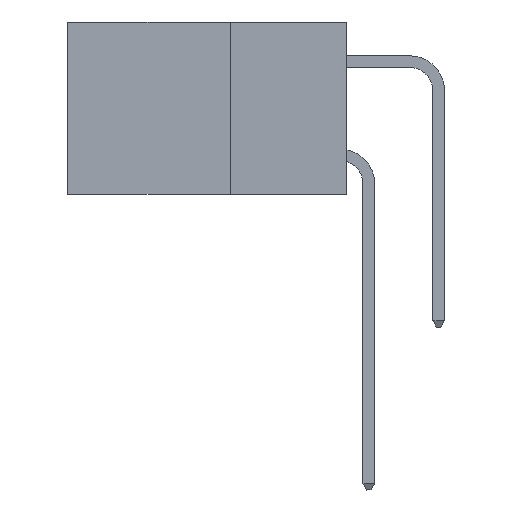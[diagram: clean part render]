
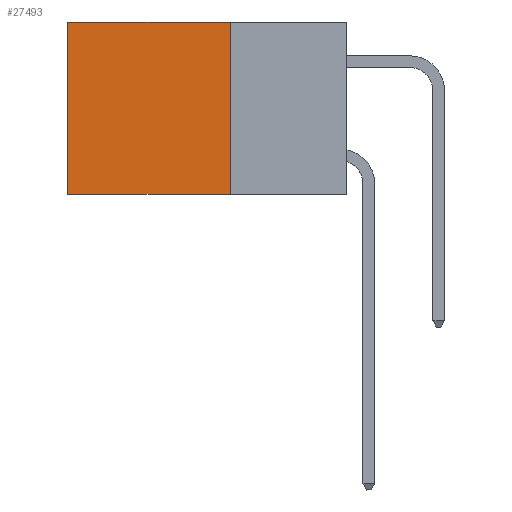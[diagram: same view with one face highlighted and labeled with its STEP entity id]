
A CAD part, left-side view. The second image highlights one B-rep face of the part: STEP entity #27493.
In plain terms, the highlighted planar face has unit normal (-1, 0, 0).
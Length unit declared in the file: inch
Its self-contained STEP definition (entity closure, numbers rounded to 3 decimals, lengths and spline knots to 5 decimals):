
#363 = VERTEX_POINT ( 'NONE', #18984 ) ;
#1046 = DIRECTION ( 'NONE',  ( 0., 1., 0. ) ) ;
#2735 = CARTESIAN_POINT ( 'NONE',  ( 0.2875, 0.25, -0.37 ) ) ;
#2800 = DIRECTION ( 'NONE',  ( 0., 0., -1. ) ) ;
#3323 = VERTEX_POINT ( 'NONE', #14393 ) ;
#4624 = EDGE_CURVE ( 'NONE', #3323, #363, #29735, .T. ) ;
#5060 = ORIENTED_EDGE ( 'NONE', *, *, #22631, .F. ) ;
#7371 = VECTOR ( 'NONE', #22149, 39.37008 ) ;
#7575 = ORIENTED_EDGE ( 'NONE', *, *, #4624, .T. ) ;
#7855 = LINE ( 'NONE', #24514, #26828 ) ;
#8529 = CARTESIAN_POINT ( 'NONE',  ( 0.2875, 0.25, 0. ) ) ;
#8904 = DIRECTION ( 'NONE',  ( 0., 0., -1. ) ) ;
#9681 = FACE_OUTER_BOUND ( 'NONE', #22427, .T. ) ;
#9846 = AXIS2_PLACEMENT_3D ( 'NONE', #18028, #20456, #2800 ) ;
#13505 = EDGE_CURVE ( 'NONE', #3323, #29063, #32188, .T. ) ;
#14393 = CARTESIAN_POINT ( 'NONE',  ( 0.2875, 0.25, 0. ) ) ;
#15270 = ORIENTED_EDGE ( 'NONE', *, *, #13505, .F. ) ;
#15815 = PLANE ( 'NONE',  #9846 ) ;
#16532 = CARTESIAN_POINT ( 'NONE',  ( 0.2875, 0.25, 0. ) ) ;
#17319 = EDGE_CURVE ( 'NONE', #363, #26262, #7855, .T. ) ;
#18028 = CARTESIAN_POINT ( 'NONE',  ( 0.2875, 0.25, 0. ) ) ;
#18984 = CARTESIAN_POINT ( 'NONE',  ( 0.2875, 0.6, 0. ) ) ;
#20323 = VECTOR ( 'NONE', #8904, 39.37008 ) ;
#20456 = DIRECTION ( 'NONE',  ( 1., 0., 0. ) ) ;
#21624 = CARTESIAN_POINT ( 'NONE',  ( 0.2875, 0.6, -0.37 ) ) ;
#22149 = DIRECTION ( 'NONE',  ( 0., 1., 0. ) ) ;
#22427 = EDGE_LOOP ( 'NONE', ( #28074, #5060, #15270, #7575 ) ) ;
#22631 = EDGE_CURVE ( 'NONE', #29063, #26262, #29069, .T. ) ;
#24514 = CARTESIAN_POINT ( 'NONE',  ( 0.2875, 0.6, 0. ) ) ;
#26262 = VERTEX_POINT ( 'NONE', #21624 ) ;
#26828 = VECTOR ( 'NONE', #29422, 39.37008 ) ;
#26984 = CARTESIAN_POINT ( 'NONE',  ( 0.2875, 0.25, -0.37 ) ) ;
#27493 = ADVANCED_FACE ( 'NONE', ( #9681 ), #15815, .F. ) ;
#28074 = ORIENTED_EDGE ( 'NONE', *, *, #17319, .T. ) ;
#29063 = VERTEX_POINT ( 'NONE', #2735 ) ;
#29069 = LINE ( 'NONE', #26984, #7371 ) ;
#29422 = DIRECTION ( 'NONE',  ( 0., 0., -1. ) ) ;
#29735 = LINE ( 'NONE', #8529, #32525 ) ;
#32188 = LINE ( 'NONE', #16532, #20323 ) ;
#32525 = VECTOR ( 'NONE', #1046, 39.37008 ) ;
